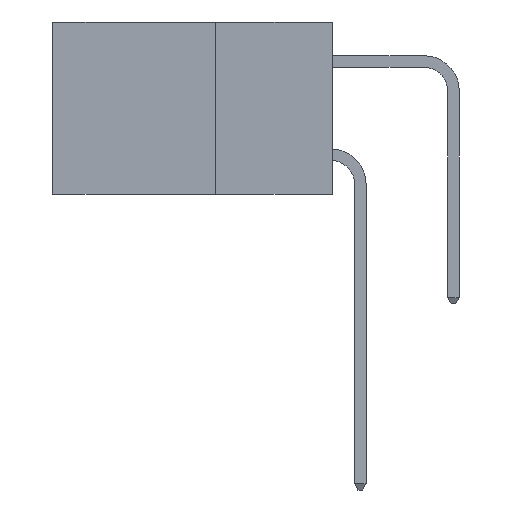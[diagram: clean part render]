
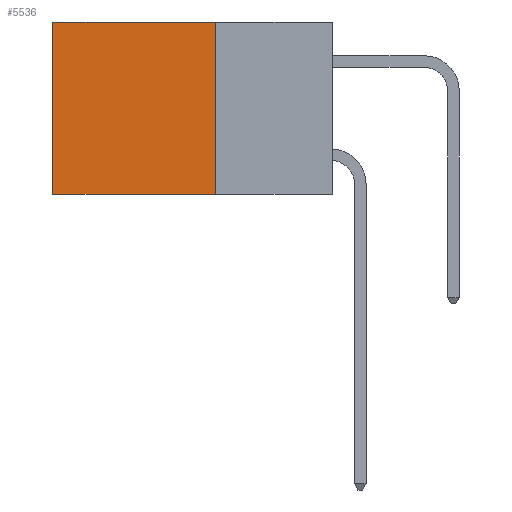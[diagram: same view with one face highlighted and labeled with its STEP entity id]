
A CAD part, left-side view. The second image highlights one B-rep face of the part: STEP entity #5536.
In plain terms, the highlighted planar face has unit normal (-1, 0, 0).
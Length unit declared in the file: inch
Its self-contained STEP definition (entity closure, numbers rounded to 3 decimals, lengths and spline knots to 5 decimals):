
#584 = VERTEX_POINT ( 'NONE', #5635 ) ;
#1320 = CARTESIAN_POINT ( 'NONE',  ( 0.2615, 0.25, -0.37 ) ) ;
#2690 = DIRECTION ( 'NONE',  ( 0., 1., 0. ) ) ;
#3225 = EDGE_CURVE ( 'NONE', #15342, #11380, #6327, .T. ) ;
#3330 = AXIS2_PLACEMENT_3D ( 'NONE', #7208, #7316, #7053 ) ;
#3866 = ORIENTED_EDGE ( 'NONE', *, *, #3225, .F. ) ;
#3901 = CARTESIAN_POINT ( 'NONE',  ( 0.2615, 0.25, 0. ) ) ;
#4396 = CARTESIAN_POINT ( 'NONE',  ( 0.2615, 0.25, 0. ) ) ;
#5536 = ADVANCED_FACE ( 'NONE', ( #14436 ), #7256, .F. ) ;
#5635 = CARTESIAN_POINT ( 'NONE',  ( 0.2615, 0.6, 0. ) ) ;
#5690 = CARTESIAN_POINT ( 'NONE',  ( 0.2615, 0.6, -0.37 ) ) ;
#6015 = VECTOR ( 'NONE', #2690, 39.37008 ) ;
#6327 = LINE ( 'NONE', #13307, #8869 ) ;
#7053 = DIRECTION ( 'NONE',  ( 0., 0., -1. ) ) ;
#7102 = DIRECTION ( 'NONE',  ( 0., 0., -1. ) ) ;
#7121 = CARTESIAN_POINT ( 'NONE',  ( 0.2615, 0.6, -0.37 ) ) ;
#7134 = LINE ( 'NONE', #11029, #14699 ) ;
#7208 = CARTESIAN_POINT ( 'NONE',  ( 0.2615, 0.25, -0.37 ) ) ;
#7209 = LINE ( 'NONE', #7121, #11130 ) ;
#7256 = PLANE ( 'NONE',  #3330 ) ;
#7316 = DIRECTION ( 'NONE',  ( 1., 0., 0. ) ) ;
#8210 = ORIENTED_EDGE ( 'NONE', *, *, #11879, .T. ) ;
#8254 = EDGE_LOOP ( 'NONE', ( #12712, #13917, #3866, #8210 ) ) ;
#8869 = VECTOR ( 'NONE', #13880, 39.37008 ) ;
#9642 = LINE ( 'NONE', #3901, #6015 ) ;
#10172 = EDGE_CURVE ( 'NONE', #584, #10810, #7209, .T. ) ;
#10810 = VERTEX_POINT ( 'NONE', #5690 ) ;
#11029 = CARTESIAN_POINT ( 'NONE',  ( 0.2615, 0.25, -0.37 ) ) ;
#11130 = VECTOR ( 'NONE', #7102, 39.37008 ) ;
#11380 = VERTEX_POINT ( 'NONE', #1320 ) ;
#11879 = EDGE_CURVE ( 'NONE', #15342, #584, #9642, .T. ) ;
#12227 = DIRECTION ( 'NONE',  ( 0., 1., 0. ) ) ;
#12712 = ORIENTED_EDGE ( 'NONE', *, *, #10172, .T. ) ;
#13307 = CARTESIAN_POINT ( 'NONE',  ( 0.2615, 0.25, -0.37 ) ) ;
#13880 = DIRECTION ( 'NONE',  ( 0., 0., -1. ) ) ;
#13917 = ORIENTED_EDGE ( 'NONE', *, *, #14194, .F. ) ;
#14194 = EDGE_CURVE ( 'NONE', #11380, #10810, #7134, .T. ) ;
#14436 = FACE_OUTER_BOUND ( 'NONE', #8254, .T. ) ;
#14699 = VECTOR ( 'NONE', #12227, 39.37008 ) ;
#15342 = VERTEX_POINT ( 'NONE', #4396 ) ;
